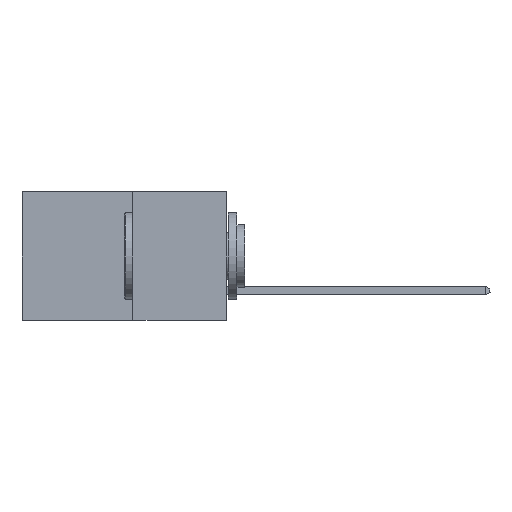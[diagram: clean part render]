
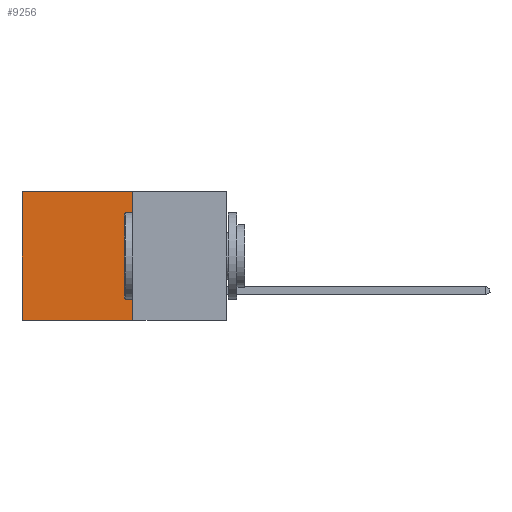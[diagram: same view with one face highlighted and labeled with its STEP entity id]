
A CAD part, left-side view. The second image highlights one B-rep face of the part: STEP entity #9256.
In plain terms, the highlighted planar face has unit normal (-1, 0, 0).
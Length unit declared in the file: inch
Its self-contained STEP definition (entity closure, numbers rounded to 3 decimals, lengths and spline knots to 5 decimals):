
#119 = DIRECTION ( 'NONE',  ( 0., 1., 0. ) ) ;
#321 = ORIENTED_EDGE ( 'NONE', *, *, #22862, .T. ) ;
#1690 = CARTESIAN_POINT ( 'NONE',  ( 0.277, 0.59, -0.37 ) ) ;
#5102 = ORIENTED_EDGE ( 'NONE', *, *, #18306, .F. ) ;
#5526 = CARTESIAN_POINT ( 'NONE',  ( 0.277, 0.27, 0. ) ) ;
#5837 = CARTESIAN_POINT ( 'NONE',  ( 0.277, 0.27, -0.37 ) ) ;
#6708 = VERTEX_POINT ( 'NONE', #19640 ) ;
#8313 = LINE ( 'NONE', #5526, #21490 ) ;
#8952 = DIRECTION ( 'NONE',  ( 1., 0., 0. ) ) ;
#9026 = VERTEX_POINT ( 'NONE', #13405 ) ;
#9256 = ADVANCED_FACE ( 'NONE', ( #14661 ), #21388, .F. ) ;
#9438 = CARTESIAN_POINT ( 'NONE',  ( 0.277, 0.59, 0. ) ) ;
#10050 = VECTOR ( 'NONE', #11947, 39.37008 ) ;
#10100 = ORIENTED_EDGE ( 'NONE', *, *, #11925, .T. ) ;
#10755 = DIRECTION ( 'NONE',  ( 0., 0., -1. ) ) ;
#11296 = DIRECTION ( 'NONE',  ( 0., 0., -1. ) ) ;
#11583 = LINE ( 'NONE', #1690, #20061 ) ;
#11925 = EDGE_CURVE ( 'NONE', #19909, #12002, #8313, .T. ) ;
#11947 = DIRECTION ( 'NONE',  ( 0., 1., 0. ) ) ;
#12002 = VERTEX_POINT ( 'NONE', #9438 ) ;
#13405 = CARTESIAN_POINT ( 'NONE',  ( 0.277, 0.27, -0.37 ) ) ;
#13506 = VECTOR ( 'NONE', #11296, 39.37008 ) ;
#14281 = CARTESIAN_POINT ( 'NONE',  ( 0.277, 0.27, -0.37 ) ) ;
#14661 = FACE_OUTER_BOUND ( 'NONE', #16976, .T. ) ;
#15417 = LINE ( 'NONE', #15526, #10050 ) ;
#15526 = CARTESIAN_POINT ( 'NONE',  ( 0.277, 0.27, -0.37 ) ) ;
#16042 = ORIENTED_EDGE ( 'NONE', *, *, #19737, .F. ) ;
#16084 = CARTESIAN_POINT ( 'NONE',  ( 0.277, 0.27, 0. ) ) ;
#16976 = EDGE_LOOP ( 'NONE', ( #321, #16042, #5102, #10100 ) ) ;
#18306 = EDGE_CURVE ( 'NONE', #19909, #9026, #18328, .T. ) ;
#18328 = LINE ( 'NONE', #5837, #13506 ) ;
#19640 = CARTESIAN_POINT ( 'NONE',  ( 0.277, 0.59, -0.37 ) ) ;
#19737 = EDGE_CURVE ( 'NONE', #9026, #6708, #15417, .T. ) ;
#19909 = VERTEX_POINT ( 'NONE', #16084 ) ;
#20061 = VECTOR ( 'NONE', #10755, 39.37008 ) ;
#21105 = AXIS2_PLACEMENT_3D ( 'NONE', #14281, #8952, #21468 ) ;
#21388 = PLANE ( 'NONE',  #21105 ) ;
#21468 = DIRECTION ( 'NONE',  ( 0., 0., -1. ) ) ;
#21490 = VECTOR ( 'NONE', #119, 39.37008 ) ;
#22862 = EDGE_CURVE ( 'NONE', #12002, #6708, #11583, .T. ) ;
